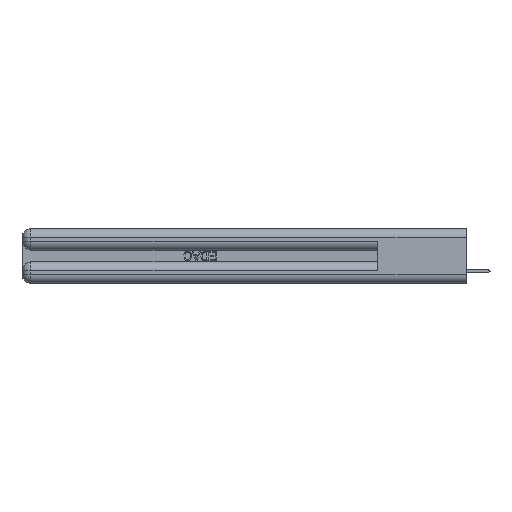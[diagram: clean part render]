
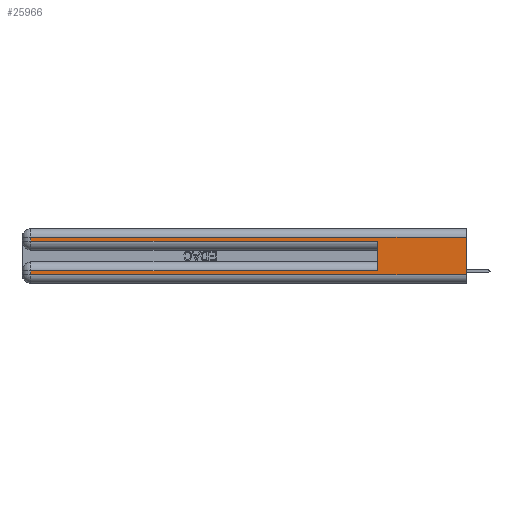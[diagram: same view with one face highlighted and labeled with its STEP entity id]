
A CAD part, left-side view. The second image highlights one B-rep face of the part: STEP entity #25966.
In plain terms, the highlighted planar face has unit normal (-1, 0, 0).
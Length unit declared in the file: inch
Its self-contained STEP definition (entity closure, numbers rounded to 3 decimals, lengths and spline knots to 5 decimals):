
#382 = VECTOR ( 'NONE', #4574, 39.37008 ) ;
#1461 = DIRECTION ( 'NONE',  ( 0., 1., 0. ) ) ;
#1981 = DIRECTION ( 'NONE',  ( 0., 0., -1. ) ) ;
#2158 = DIRECTION ( 'NONE',  ( 1., 0., 0. ) ) ;
#2478 = CARTESIAN_POINT ( 'NONE',  ( 0., 0., 0.37 ) ) ;
#4574 = DIRECTION ( 'NONE',  ( 0., 0., -1. ) ) ;
#6345 = VECTOR ( 'NONE', #42579, 39.37008 ) ;
#6405 = VECTOR ( 'NONE', #30056, 39.37008 ) ;
#7977 = DIRECTION ( 'NONE',  ( 0., 0., 1. ) ) ;
#8809 = EDGE_CURVE ( 'NONE', #9484, #14706, #16444, .T. ) ;
#9343 = CARTESIAN_POINT ( 'NONE',  ( 0., 0., 0.06 ) ) ;
#9484 = VERTEX_POINT ( 'NONE', #19677 ) ;
#10343 = VERTEX_POINT ( 'NONE', #13688 ) ;
#11151 = CARTESIAN_POINT ( 'NONE',  ( 0., 0., 0.31 ) ) ;
#11154 = CARTESIAN_POINT ( 'NONE',  ( 0., 0., 0.37 ) ) ;
#11241 = VERTEX_POINT ( 'NONE', #9343 ) ;
#12097 = EDGE_CURVE ( 'NONE', #43845, #10343, #42331, .T. ) ;
#13206 = VECTOR ( 'NONE', #1461, 39.37008 ) ;
#13688 = CARTESIAN_POINT ( 'NONE',  ( 0., 2.94, 0.31 ) ) ;
#14300 = FACE_OUTER_BOUND ( 'NONE', #48541, .T. ) ;
#14706 = VERTEX_POINT ( 'NONE', #37379 ) ;
#16444 = LINE ( 'NONE', #41059, #6405 ) ;
#17772 = VECTOR ( 'NONE', #18789, 39.37008 ) ;
#18789 = DIRECTION ( 'NONE',  ( 0., 0., -1. ) ) ;
#19465 = LINE ( 'NONE', #11154, #17772 ) ;
#19677 = CARTESIAN_POINT ( 'NONE',  ( 0., 2.94, 0.285 ) ) ;
#20325 = EDGE_CURVE ( 'NONE', #26743, #32416, #40894, .T. ) ;
#21323 = ORIENTED_EDGE ( 'NONE', *, *, #8809, .T. ) ;
#21998 = EDGE_CURVE ( 'NONE', #32416, #11241, #28250, .T. ) ;
#22708 = ORIENTED_EDGE ( 'NONE', *, *, #37484, .T. ) ;
#23675 = CARTESIAN_POINT ( 'NONE',  ( 0., 2.94, 0.37 ) ) ;
#25210 = DIRECTION ( 'NONE',  ( 0., 0., -1. ) ) ;
#25966 = ADVANCED_FACE ( 'NONE', ( #14300 ), #39028, .F. ) ;
#26126 = ORIENTED_EDGE ( 'NONE', *, *, #21998, .T. ) ;
#26648 = EDGE_CURVE ( 'NONE', #43845, #11241, #19465, .T. ) ;
#26743 = VERTEX_POINT ( 'NONE', #48674 ) ;
#28250 = LINE ( 'NONE', #35582, #6345 ) ;
#30056 = DIRECTION ( 'NONE',  ( 0., -1., 0. ) ) ;
#30323 = VECTOR ( 'NONE', #25210, 39.37008 ) ;
#30887 = ORIENTED_EDGE ( 'NONE', *, *, #12097, .T. ) ;
#30970 = ORIENTED_EDGE ( 'NONE', *, *, #26648, .F. ) ;
#31181 = ORIENTED_EDGE ( 'NONE', *, *, #20325, .T. ) ;
#31780 = CARTESIAN_POINT ( 'NONE',  ( 0., 2.94, 0.06 ) ) ;
#32028 = LINE ( 'NONE', #41949, #45155 ) ;
#32416 = VERTEX_POINT ( 'NONE', #31780 ) ;
#32954 = CARTESIAN_POINT ( 'NONE',  ( 0., 0., 0.31 ) ) ;
#33912 = AXIS2_PLACEMENT_3D ( 'NONE', #2478, #2158, #1981 ) ;
#34023 = ORIENTED_EDGE ( 'NONE', *, *, #47595, .F. ) ;
#34914 = CARTESIAN_POINT ( 'NONE',  ( 0., 0.6, 0.085 ) ) ;
#35582 = CARTESIAN_POINT ( 'NONE',  ( 0., 0., 0.06 ) ) ;
#35963 = DIRECTION ( 'NONE',  ( 0., 1., 0. ) ) ;
#36253 = ORIENTED_EDGE ( 'NONE', *, *, #45491, .T. ) ;
#37379 = CARTESIAN_POINT ( 'NONE',  ( 0., 0.6, 0.285 ) ) ;
#37484 = EDGE_CURVE ( 'NONE', #44525, #26743, #42545, .T. ) ;
#39028 = PLANE ( 'NONE',  #33912 ) ;
#40894 = LINE ( 'NONE', #23675, #382 ) ;
#40901 = CARTESIAN_POINT ( 'NONE',  ( 0., 2.94, 0.37 ) ) ;
#41059 = CARTESIAN_POINT ( 'NONE',  ( 0., 0., 0.285 ) ) ;
#41949 = CARTESIAN_POINT ( 'NONE',  ( 0., 0.6, 0.145 ) ) ;
#42331 = LINE ( 'NONE', #11151, #13206 ) ;
#42545 = LINE ( 'NONE', #43104, #45000 ) ;
#42579 = DIRECTION ( 'NONE',  ( 0., -1., 0. ) ) ;
#43104 = CARTESIAN_POINT ( 'NONE',  ( 0., 0., 0.085 ) ) ;
#43845 = VERTEX_POINT ( 'NONE', #32954 ) ;
#44525 = VERTEX_POINT ( 'NONE', #34914 ) ;
#45000 = VECTOR ( 'NONE', #35963, 39.37008 ) ;
#45155 = VECTOR ( 'NONE', #7977, 39.37008 ) ;
#45491 = EDGE_CURVE ( 'NONE', #10343, #9484, #47598, .T. ) ;
#47595 = EDGE_CURVE ( 'NONE', #44525, #14706, #32028, .T. ) ;
#47598 = LINE ( 'NONE', #40901, #30323 ) ;
#48541 = EDGE_LOOP ( 'NONE', ( #30970, #30887, #36253, #21323, #34023, #22708, #31181, #26126 ) ) ;
#48674 = CARTESIAN_POINT ( 'NONE',  ( 0., 2.94, 0.085 ) ) ;
